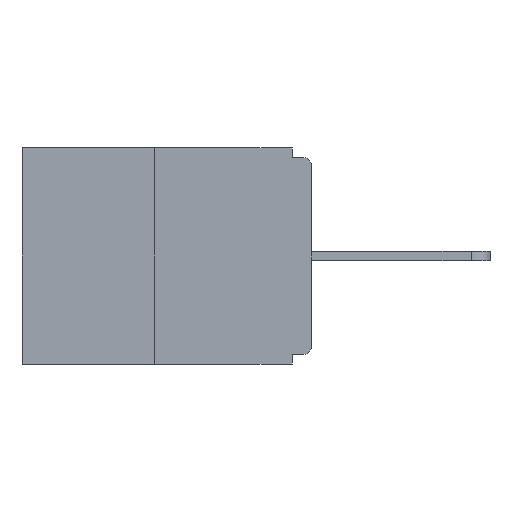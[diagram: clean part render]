
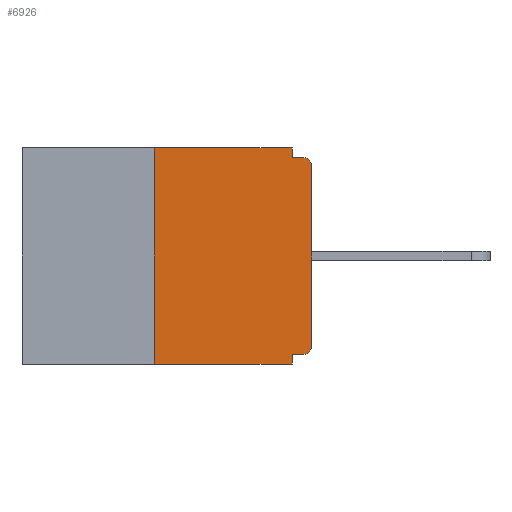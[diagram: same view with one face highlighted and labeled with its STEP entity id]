
A CAD part, left-side view. The second image highlights one B-rep face of the part: STEP entity #6926.
In plain terms, the highlighted planar face has unit normal (-1, 0, 0).
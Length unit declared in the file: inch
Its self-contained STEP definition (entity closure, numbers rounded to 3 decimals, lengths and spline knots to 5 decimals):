
#116 = EDGE_CURVE ( 'NONE', #8865, #3749, #10065, .T. ) ;
#280 = CIRCLE ( 'NONE', #6195, 0.015 ) ;
#939 = ORIENTED_EDGE ( 'NONE', *, *, #12357, .T. ) ;
#1094 = LINE ( 'NONE', #9153, #7326 ) ;
#1338 = ORIENTED_EDGE ( 'NONE', *, *, #11393, .F. ) ;
#1564 = EDGE_CURVE ( 'NONE', #8381, #14790, #2685, .T. ) ;
#1737 = DIRECTION ( 'NONE',  ( 0., 0., 1. ) ) ;
#1763 = VERTEX_POINT ( 'NONE', #10280 ) ;
#2299 = ORIENTED_EDGE ( 'NONE', *, *, #10883, .F. ) ;
#2595 = FACE_OUTER_BOUND ( 'NONE', #3016, .T. ) ;
#2685 = CIRCLE ( 'NONE', #9401, 0.015 ) ;
#2690 = VECTOR ( 'NONE', #9736, 39.37008 ) ;
#2909 = CARTESIAN_POINT ( 'NONE',  ( 0., 0.25, -0.343 ) ) ;
#3016 = EDGE_LOOP ( 'NONE', ( #8500, #2299, #15445, #10034, #10409, #13490, #939, #13845, #1338, #8320 ) ) ;
#3073 = VERTEX_POINT ( 'NONE', #11726 ) ;
#3076 = LINE ( 'NONE', #6061, #2690 ) ;
#3480 = VERTEX_POINT ( 'NONE', #2909 ) ;
#3749 = VERTEX_POINT ( 'NONE', #15087 ) ;
#3917 = DIRECTION ( 'NONE',  ( -1., 0., 0. ) ) ;
#3938 = CARTESIAN_POINT ( 'NONE',  ( 0., 0.031, -0.343 ) ) ;
#4180 = VECTOR ( 'NONE', #5978, 39.37008 ) ;
#4232 = EDGE_CURVE ( 'NONE', #3480, #14335, #9249, .T. ) ;
#5018 = VECTOR ( 'NONE', #11951, 39.37008 ) ;
#5742 = EDGE_CURVE ( 'NONE', #3073, #12542, #280, .T. ) ;
#5978 = DIRECTION ( 'NONE',  ( 0., 0., -1. ) ) ;
#6019 = VECTOR ( 'NONE', #12225, 39.37008 ) ;
#6061 = CARTESIAN_POINT ( 'NONE',  ( 0., 0., -0.015 ) ) ;
#6195 = AXIS2_PLACEMENT_3D ( 'NONE', #6783, #6849, #6842 ) ;
#6198 = DIRECTION ( 'NONE',  ( 0., 1., 0. ) ) ;
#6374 = PLANE ( 'NONE',  #11448 ) ;
#6783 = CARTESIAN_POINT ( 'NONE',  ( 0., 0.015, -0.313 ) ) ;
#6801 = CARTESIAN_POINT ( 'NONE',  ( 0., 0.46, 0. ) ) ;
#6810 = VECTOR ( 'NONE', #11947, 39.37008 ) ;
#6842 = DIRECTION ( 'NONE',  ( 0., 0., -1. ) ) ;
#6849 = DIRECTION ( 'NONE',  ( -1., 0., 0. ) ) ;
#6926 = ADVANCED_FACE ( 'NONE', ( #2595 ), #6374, .F. ) ;
#7245 = CARTESIAN_POINT ( 'NONE',  ( 0., 0.25, 0. ) ) ;
#7326 = VECTOR ( 'NONE', #1737, 39.37008 ) ;
#7481 = LINE ( 'NONE', #13130, #4180 ) ;
#7941 = LINE ( 'NONE', #7245, #14581 ) ;
#8320 = ORIENTED_EDGE ( 'NONE', *, *, #15218, .F. ) ;
#8381 = VERTEX_POINT ( 'NONE', #9112 ) ;
#8500 = ORIENTED_EDGE ( 'NONE', *, *, #116, .F. ) ;
#8865 = VERTEX_POINT ( 'NONE', #9150 ) ;
#9112 = CARTESIAN_POINT ( 'NONE',  ( 0., 0., -0.03 ) ) ;
#9150 = CARTESIAN_POINT ( 'NONE',  ( 0., 0.25, 0. ) ) ;
#9153 = CARTESIAN_POINT ( 'NONE',  ( 0., 0., 0. ) ) ;
#9249 = LINE ( 'NONE', #10314, #6019 ) ;
#9401 = AXIS2_PLACEMENT_3D ( 'NONE', #10508, #3917, #10404 ) ;
#9542 = CARTESIAN_POINT ( 'NONE',  ( 0., 0., -0.313 ) ) ;
#9736 = DIRECTION ( 'NONE',  ( 0., -1., 0. ) ) ;
#9948 = CARTESIAN_POINT ( 'NONE',  ( 0., 0.031, -0.015 ) ) ;
#10034 = ORIENTED_EDGE ( 'NONE', *, *, #14073, .F. ) ;
#10065 = LINE ( 'NONE', #14802, #6810 ) ;
#10280 = CARTESIAN_POINT ( 'NONE',  ( 0., 0.031, -0.328 ) ) ;
#10314 = CARTESIAN_POINT ( 'NONE',  ( 0., 0.46, -0.343 ) ) ;
#10365 = EDGE_CURVE ( 'NONE', #3073, #1763, #15298, .T. ) ;
#10404 = DIRECTION ( 'NONE',  ( 0., 0., -1. ) ) ;
#10409 = ORIENTED_EDGE ( 'NONE', *, *, #10365, .F. ) ;
#10508 = CARTESIAN_POINT ( 'NONE',  ( 0., 0.015, -0.03 ) ) ;
#10883 = EDGE_CURVE ( 'NONE', #3480, #8865, #7941, .T. ) ;
#11393 = EDGE_CURVE ( 'NONE', #13084, #14790, #3076, .T. ) ;
#11448 = AXIS2_PLACEMENT_3D ( 'NONE', #6801, #14902, #14898 ) ;
#11726 = CARTESIAN_POINT ( 'NONE',  ( 0., 0.015, -0.328 ) ) ;
#11901 = VECTOR ( 'NONE', #6198, 39.37008 ) ;
#11947 = DIRECTION ( 'NONE',  ( 0., -1., 0. ) ) ;
#11951 = DIRECTION ( 'NONE',  ( 0., 0., -1. ) ) ;
#12225 = DIRECTION ( 'NONE',  ( 0., -1., 0. ) ) ;
#12357 = EDGE_CURVE ( 'NONE', #12542, #8381, #1094, .T. ) ;
#12542 = VERTEX_POINT ( 'NONE', #9542 ) ;
#13084 = VERTEX_POINT ( 'NONE', #9948 ) ;
#13130 = CARTESIAN_POINT ( 'NONE',  ( 0., 0.031, -0.343 ) ) ;
#13490 = ORIENTED_EDGE ( 'NONE', *, *, #5742, .T. ) ;
#13845 = ORIENTED_EDGE ( 'NONE', *, *, #1564, .T. ) ;
#14073 = EDGE_CURVE ( 'NONE', #1763, #14335, #7481, .T. ) ;
#14173 = LINE ( 'NONE', #14235, #5018 ) ;
#14235 = CARTESIAN_POINT ( 'NONE',  ( 0., 0.031, 0. ) ) ;
#14335 = VERTEX_POINT ( 'NONE', #3938 ) ;
#14434 = CARTESIAN_POINT ( 'NONE',  ( 0., 0., -0.328 ) ) ;
#14581 = VECTOR ( 'NONE', #15456, 39.37008 ) ;
#14790 = VERTEX_POINT ( 'NONE', #15547 ) ;
#14802 = CARTESIAN_POINT ( 'NONE',  ( 0., 0.46, 0. ) ) ;
#14898 = DIRECTION ( 'NONE',  ( 0., 0., -1. ) ) ;
#14902 = DIRECTION ( 'NONE',  ( 1., 0., 0. ) ) ;
#15087 = CARTESIAN_POINT ( 'NONE',  ( 0., 0.031, 0. ) ) ;
#15218 = EDGE_CURVE ( 'NONE', #3749, #13084, #14173, .T. ) ;
#15298 = LINE ( 'NONE', #14434, #11901 ) ;
#15445 = ORIENTED_EDGE ( 'NONE', *, *, #4232, .T. ) ;
#15456 = DIRECTION ( 'NONE',  ( 0., 0., 1. ) ) ;
#15547 = CARTESIAN_POINT ( 'NONE',  ( 0., 0.015, -0.015 ) ) ;
